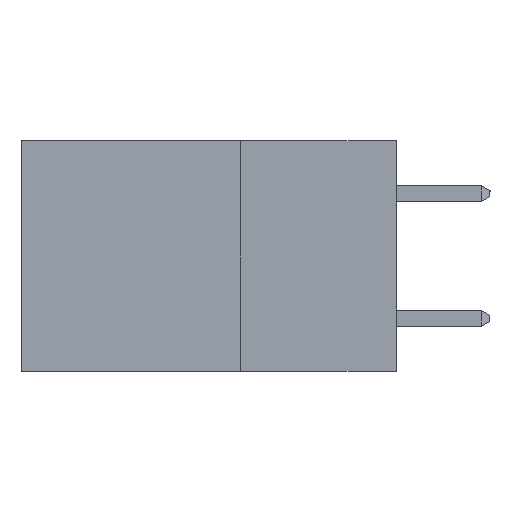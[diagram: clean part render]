
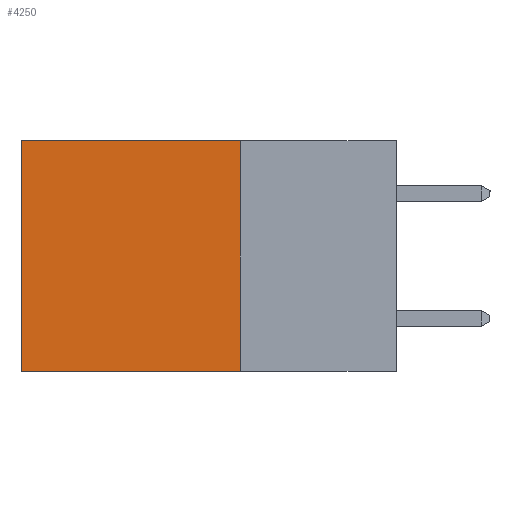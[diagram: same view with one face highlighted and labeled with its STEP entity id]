
A CAD part, left-side view. The second image highlights one B-rep face of the part: STEP entity #4250.
In plain terms, the highlighted planar face has unit normal (-1, 0, 0).
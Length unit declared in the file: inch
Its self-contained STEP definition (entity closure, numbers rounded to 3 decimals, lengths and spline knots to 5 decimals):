
#573 = DIRECTION ( 'NONE',  ( 0., 1., 0. ) ) ;
#610 = DIRECTION ( 'NONE',  ( 0., 0., -1. ) ) ;
#643 = VERTEX_POINT ( 'NONE', #7490 ) ;
#1259 = DIRECTION ( 'NONE',  ( 0., 0., -1. ) ) ;
#1736 = EDGE_LOOP ( 'NONE', ( #6178, #11985, #4171, #1749 ) ) ;
#1749 = ORIENTED_EDGE ( 'NONE', *, *, #8068, .T. ) ;
#2615 = PLANE ( 'NONE',  #6754 ) ;
#2664 = DIRECTION ( 'NONE',  ( 0., 0., -1. ) ) ;
#2738 = VECTOR ( 'NONE', #2664, 39.37008 ) ;
#3967 = CARTESIAN_POINT ( 'NONE',  ( 0.2615, 0.25, -0.37 ) ) ;
#4171 = ORIENTED_EDGE ( 'NONE', *, *, #7788, .F. ) ;
#4250 = ADVANCED_FACE ( 'NONE', ( #8727 ), #2615, .F. ) ;
#4334 = DIRECTION ( 'NONE',  ( 0., 1., 0. ) ) ;
#4405 = LINE ( 'NONE', #10367, #11992 ) ;
#5078 = CARTESIAN_POINT ( 'NONE',  ( 0.2615, 0.25, -0.37 ) ) ;
#6178 = ORIENTED_EDGE ( 'NONE', *, *, #8890, .T. ) ;
#6754 = AXIS2_PLACEMENT_3D ( 'NONE', #3967, #7349, #1259 ) ;
#7249 = VERTEX_POINT ( 'NONE', #5078 ) ;
#7349 = DIRECTION ( 'NONE',  ( 1., 0., 0. ) ) ;
#7391 = EDGE_CURVE ( 'NONE', #7249, #10934, #11529, .T. ) ;
#7490 = CARTESIAN_POINT ( 'NONE',  ( 0.2615, 0.6, 0. ) ) ;
#7788 = EDGE_CURVE ( 'NONE', #11229, #7249, #11285, .T. ) ;
#8000 = LINE ( 'NONE', #11481, #12018 ) ;
#8068 = EDGE_CURVE ( 'NONE', #11229, #643, #4405, .T. ) ;
#8727 = FACE_OUTER_BOUND ( 'NONE', #1736, .T. ) ;
#8890 = EDGE_CURVE ( 'NONE', #643, #10934, #8000, .T. ) ;
#9442 = CARTESIAN_POINT ( 'NONE',  ( 0.2615, 0.25, 0. ) ) ;
#9805 = CARTESIAN_POINT ( 'NONE',  ( 0.2615, 0.25, -0.37 ) ) ;
#10367 = CARTESIAN_POINT ( 'NONE',  ( 0.2615, 0.25, 0. ) ) ;
#10934 = VERTEX_POINT ( 'NONE', #14352 ) ;
#11229 = VERTEX_POINT ( 'NONE', #9442 ) ;
#11285 = LINE ( 'NONE', #9805, #2738 ) ;
#11481 = CARTESIAN_POINT ( 'NONE',  ( 0.2615, 0.6, -0.37 ) ) ;
#11529 = LINE ( 'NONE', #13056, #13016 ) ;
#11985 = ORIENTED_EDGE ( 'NONE', *, *, #7391, .F. ) ;
#11992 = VECTOR ( 'NONE', #573, 39.37008 ) ;
#12018 = VECTOR ( 'NONE', #610, 39.37008 ) ;
#13016 = VECTOR ( 'NONE', #4334, 39.37008 ) ;
#13056 = CARTESIAN_POINT ( 'NONE',  ( 0.2615, 0.25, -0.37 ) ) ;
#14352 = CARTESIAN_POINT ( 'NONE',  ( 0.2615, 0.6, -0.37 ) ) ;
